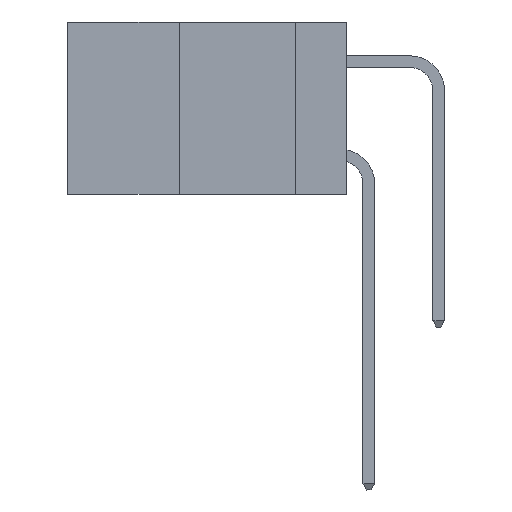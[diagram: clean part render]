
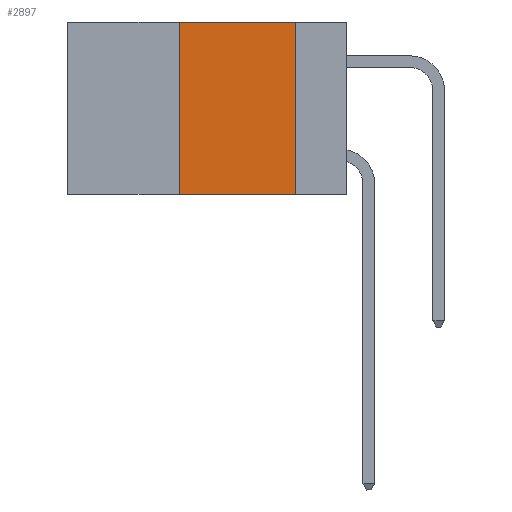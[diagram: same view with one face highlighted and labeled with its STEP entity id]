
A CAD part, left-side view. The second image highlights one B-rep face of the part: STEP entity #2897.
In plain terms, the highlighted planar face has unit normal (-1, 0, 0).
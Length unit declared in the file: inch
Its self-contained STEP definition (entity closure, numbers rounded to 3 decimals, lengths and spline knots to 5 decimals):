
#448 = AXIS2_PLACEMENT_3D ( 'NONE', #8292, #8709, #8080 ) ;
#1129 = CARTESIAN_POINT ( 'NONE',  ( 0., 0.36, -0.37 ) ) ;
#1176 = VECTOR ( 'NONE', #5779, 39.37008 ) ;
#1197 = DIRECTION ( 'NONE',  ( 0., 0., 1. ) ) ;
#1988 = ORIENTED_EDGE ( 'NONE', *, *, #6313, .F. ) ;
#2025 = LINE ( 'NONE', #4794, #10107 ) ;
#2181 = ORIENTED_EDGE ( 'NONE', *, *, #6131, .F. ) ;
#2259 = ORIENTED_EDGE ( 'NONE', *, *, #7221, .F. ) ;
#2897 = ADVANCED_FACE ( 'NONE', ( #6685 ), #8051, .F. ) ;
#3038 = DIRECTION ( 'NONE',  ( 0., 0., -1. ) ) ;
#4613 = LINE ( 'NONE', #7948, #1176 ) ;
#4794 = CARTESIAN_POINT ( 'NONE',  ( 0., 0.6, 0. ) ) ;
#5019 = CARTESIAN_POINT ( 'NONE',  ( 0., 0.36, 0. ) ) ;
#5237 = EDGE_LOOP ( 'NONE', ( #2259, #2181, #1988, #11255 ) ) ;
#5248 = CARTESIAN_POINT ( 'NONE',  ( 0., 0.11, 0. ) ) ;
#5403 = CARTESIAN_POINT ( 'NONE',  ( 0., 0.11, 0. ) ) ;
#5434 = VECTOR ( 'NONE', #1197, 39.37008 ) ;
#5779 = DIRECTION ( 'NONE',  ( 0., -1., 0. ) ) ;
#6071 = VERTEX_POINT ( 'NONE', #12724 ) ;
#6087 = LINE ( 'NONE', #5019, #5434 ) ;
#6130 = EDGE_CURVE ( 'NONE', #9649, #8421, #4613, .T. ) ;
#6131 = EDGE_CURVE ( 'NONE', #6071, #12613, #2025, .T. ) ;
#6313 = EDGE_CURVE ( 'NONE', #9649, #6071, #6087, .T. ) ;
#6577 = CARTESIAN_POINT ( 'NONE',  ( 0., 0.11, -0.37 ) ) ;
#6685 = FACE_OUTER_BOUND ( 'NONE', #5237, .T. ) ;
#7221 = EDGE_CURVE ( 'NONE', #12613, #8421, #12751, .T. ) ;
#7588 = VECTOR ( 'NONE', #3038, 39.37008 ) ;
#7948 = CARTESIAN_POINT ( 'NONE',  ( 0., 0.6, -0.37 ) ) ;
#8051 = PLANE ( 'NONE',  #448 ) ;
#8080 = DIRECTION ( 'NONE',  ( 0., 0., -1. ) ) ;
#8292 = CARTESIAN_POINT ( 'NONE',  ( 0., 0.6, 0. ) ) ;
#8421 = VERTEX_POINT ( 'NONE', #6577 ) ;
#8709 = DIRECTION ( 'NONE',  ( 1., 0., 0. ) ) ;
#9649 = VERTEX_POINT ( 'NONE', #1129 ) ;
#10107 = VECTOR ( 'NONE', #10901, 39.37008 ) ;
#10901 = DIRECTION ( 'NONE',  ( 0., -1., 0. ) ) ;
#11255 = ORIENTED_EDGE ( 'NONE', *, *, #6130, .T. ) ;
#12613 = VERTEX_POINT ( 'NONE', #5248 ) ;
#12724 = CARTESIAN_POINT ( 'NONE',  ( 0., 0.36, 0. ) ) ;
#12751 = LINE ( 'NONE', #5403, #7588 ) ;
